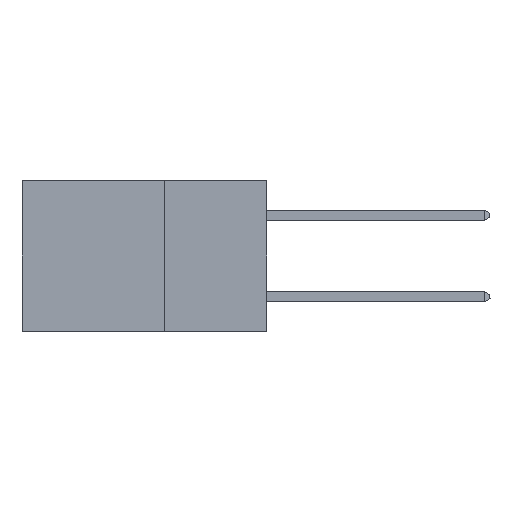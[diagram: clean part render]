
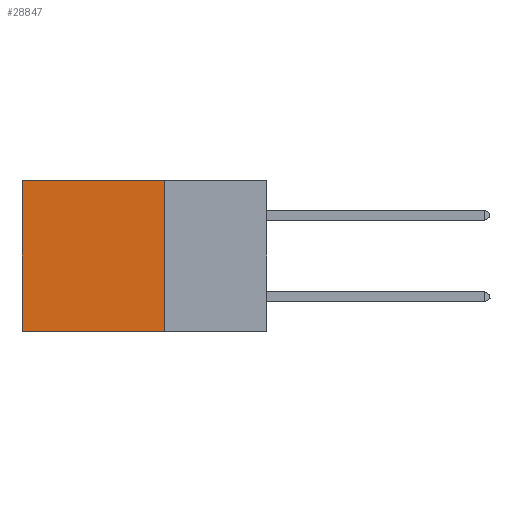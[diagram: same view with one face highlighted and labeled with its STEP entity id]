
A CAD part, left-side view. The second image highlights one B-rep face of the part: STEP entity #28847.
In plain terms, the highlighted planar face has unit normal (-1, 0, 0).
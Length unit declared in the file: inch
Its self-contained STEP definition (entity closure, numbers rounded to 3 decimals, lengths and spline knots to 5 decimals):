
#2134 = ORIENTED_EDGE ( 'NONE', *, *, #9933, .T. ) ;
#3042 = LINE ( 'NONE', #4024, #4866 ) ;
#3309 = VERTEX_POINT ( 'NONE', #19870 ) ;
#3615 = ORIENTED_EDGE ( 'NONE', *, *, #18274, .F. ) ;
#4024 = CARTESIAN_POINT ( 'NONE',  ( 0.2875, 0.25, 0. ) ) ;
#4076 = AXIS2_PLACEMENT_3D ( 'NONE', #17490, #31225, #14392 ) ;
#4491 = DIRECTION ( 'NONE',  ( 0., 0., -1. ) ) ;
#4866 = VECTOR ( 'NONE', #15798, 39.37008 ) ;
#5053 = DIRECTION ( 'NONE',  ( 0., 1., 0. ) ) ;
#5302 = CARTESIAN_POINT ( 'NONE',  ( 0.2875, 0.25, -0.37 ) ) ;
#5403 = DIRECTION ( 'NONE',  ( 0., 0., -1. ) ) ;
#5908 = CARTESIAN_POINT ( 'NONE',  ( 0.2875, 0.25, -0.37 ) ) ;
#7545 = VERTEX_POINT ( 'NONE', #5908 ) ;
#8872 = ORIENTED_EDGE ( 'NONE', *, *, #36200, .T. ) ;
#9933 = EDGE_CURVE ( 'NONE', #34795, #10838, #27776, .T. ) ;
#10838 = VERTEX_POINT ( 'NONE', #26105 ) ;
#14160 = PLANE ( 'NONE',  #4076 ) ;
#14392 = DIRECTION ( 'NONE',  ( 0., 0., -1. ) ) ;
#15405 = EDGE_LOOP ( 'NONE', ( #2134, #3615, #28059, #8872 ) ) ;
#15553 = LINE ( 'NONE', #19113, #16893 ) ;
#15798 = DIRECTION ( 'NONE',  ( 0., 1., 0. ) ) ;
#16893 = VECTOR ( 'NONE', #4491, 39.37008 ) ;
#17015 = VECTOR ( 'NONE', #5053, 39.37008 ) ;
#17490 = CARTESIAN_POINT ( 'NONE',  ( 0.2875, 0.25, 0. ) ) ;
#17956 = VECTOR ( 'NONE', #5403, 39.37008 ) ;
#18274 = EDGE_CURVE ( 'NONE', #7545, #10838, #32148, .T. ) ;
#19113 = CARTESIAN_POINT ( 'NONE',  ( 0.2875, 0.25, 0. ) ) ;
#19705 = EDGE_CURVE ( 'NONE', #3309, #7545, #15553, .T. ) ;
#19870 = CARTESIAN_POINT ( 'NONE',  ( 0.2875, 0.25, 0. ) ) ;
#21649 = FACE_OUTER_BOUND ( 'NONE', #15405, .T. ) ;
#25410 = CARTESIAN_POINT ( 'NONE',  ( 0.2875, 0.6, 0. ) ) ;
#26105 = CARTESIAN_POINT ( 'NONE',  ( 0.2875, 0.6, -0.37 ) ) ;
#27776 = LINE ( 'NONE', #25410, #17956 ) ;
#28059 = ORIENTED_EDGE ( 'NONE', *, *, #19705, .F. ) ;
#28847 = ADVANCED_FACE ( 'NONE', ( #21649 ), #14160, .F. ) ;
#30706 = CARTESIAN_POINT ( 'NONE',  ( 0.2875, 0.6, 0. ) ) ;
#31225 = DIRECTION ( 'NONE',  ( 1., 0., 0. ) ) ;
#32148 = LINE ( 'NONE', #5302, #17015 ) ;
#34795 = VERTEX_POINT ( 'NONE', #30706 ) ;
#36200 = EDGE_CURVE ( 'NONE', #3309, #34795, #3042, .T. ) ;
